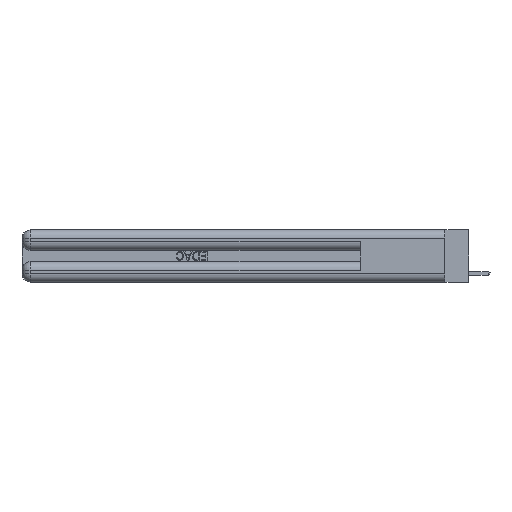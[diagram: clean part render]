
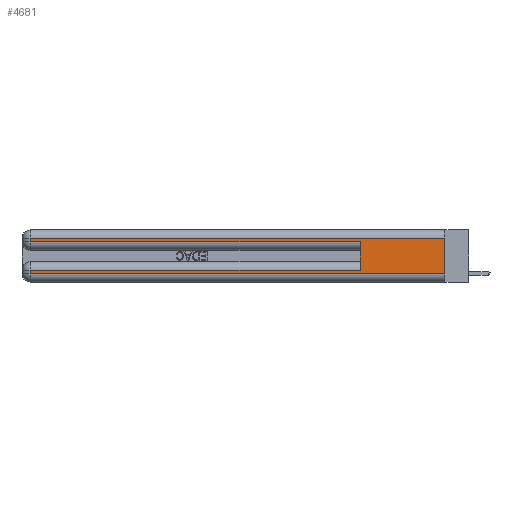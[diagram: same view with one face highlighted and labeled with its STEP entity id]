
A CAD part, left-side view. The second image highlights one B-rep face of the part: STEP entity #4681.
In plain terms, the highlighted planar face has unit normal (-1, 0, 0).
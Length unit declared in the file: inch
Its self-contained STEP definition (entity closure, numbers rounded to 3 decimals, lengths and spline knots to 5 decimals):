
#1505 = DIRECTION ( 'NONE',  ( 0., 0., -1. ) ) ;
#1712 = ORIENTED_EDGE ( 'NONE', *, *, #9419, .F. ) ;
#2761 = VECTOR ( 'NONE', #33430, 39.37008 ) ;
#2908 = DIRECTION ( 'NONE',  ( 0., 0., 1. ) ) ;
#3691 = EDGE_CURVE ( 'NONE', #10057, #9329, #4144, .T. ) ;
#4144 = LINE ( 'NONE', #16697, #21500 ) ;
#4260 = EDGE_CURVE ( 'NONE', #27985, #23001, #7281, .T. ) ;
#4681 = ADVANCED_FACE ( 'NONE', ( #18136 ), #33951, .F. ) ;
#5037 = ORIENTED_EDGE ( 'NONE', *, *, #18744, .T. ) ;
#5178 = ORIENTED_EDGE ( 'NONE', *, *, #24509, .F. ) ;
#6189 = LINE ( 'NONE', #11609, #26545 ) ;
#6500 = LINE ( 'NONE', #22339, #14391 ) ;
#7015 = AXIS2_PLACEMENT_3D ( 'NONE', #23599, #26409, #9858 ) ;
#7079 = DIRECTION ( 'NONE',  ( 0., -1., 0. ) ) ;
#7281 = LINE ( 'NONE', #24003, #27173 ) ;
#7609 = EDGE_CURVE ( 'NONE', #34385, #10057, #6500, .T. ) ;
#7647 = ORIENTED_EDGE ( 'NONE', *, *, #22046, .T. ) ;
#7881 = VECTOR ( 'NONE', #7079, 39.37008 ) ;
#9329 = VERTEX_POINT ( 'NONE', #12242 ) ;
#9419 = EDGE_CURVE ( 'NONE', #34385, #13860, #34396, .T. ) ;
#9858 = DIRECTION ( 'NONE',  ( 0., 0., -1. ) ) ;
#9875 = CARTESIAN_POINT ( 'NONE',  ( 0., 0., 0.06 ) ) ;
#9883 = CARTESIAN_POINT ( 'NONE',  ( 0., 2.94, 0.31 ) ) ;
#10057 = VERTEX_POINT ( 'NONE', #24075 ) ;
#10427 = DIRECTION ( 'NONE',  ( 0., 0., -1. ) ) ;
#11609 = CARTESIAN_POINT ( 'NONE',  ( 0., 0., 0.285 ) ) ;
#11956 = DIRECTION ( 'NONE',  ( 0., -1., 0. ) ) ;
#12094 = VERTEX_POINT ( 'NONE', #33825 ) ;
#12242 = CARTESIAN_POINT ( 'NONE',  ( 0., 2.94, 0.06 ) ) ;
#13860 = VERTEX_POINT ( 'NONE', #17883 ) ;
#14391 = VECTOR ( 'NONE', #33022, 39.37008 ) ;
#14629 = LINE ( 'NONE', #31311, #2761 ) ;
#15345 = LINE ( 'NONE', #20999, #15870 ) ;
#15870 = VECTOR ( 'NONE', #23285, 39.37008 ) ;
#16697 = CARTESIAN_POINT ( 'NONE',  ( 0., 2.94, 0.37 ) ) ;
#17404 = ORIENTED_EDGE ( 'NONE', *, *, #3691, .T. ) ;
#17883 = CARTESIAN_POINT ( 'NONE',  ( 0., 0.6, 0.285 ) ) ;
#18136 = FACE_OUTER_BOUND ( 'NONE', #26301, .T. ) ;
#18744 = EDGE_CURVE ( 'NONE', #12094, #27985, #14629, .T. ) ;
#18860 = ORIENTED_EDGE ( 'NONE', *, *, #34357, .T. ) ;
#19418 = CARTESIAN_POINT ( 'NONE',  ( 0., 0., 0.06 ) ) ;
#20696 = VECTOR ( 'NONE', #2908, 39.37008 ) ;
#20999 = CARTESIAN_POINT ( 'NONE',  ( 0., 0., 0.37 ) ) ;
#21500 = VECTOR ( 'NONE', #1505, 39.37008 ) ;
#22046 = EDGE_CURVE ( 'NONE', #9329, #27712, #34138, .T. ) ;
#22339 = CARTESIAN_POINT ( 'NONE',  ( 0., 0., 0.085 ) ) ;
#23001 = VERTEX_POINT ( 'NONE', #29271 ) ;
#23285 = DIRECTION ( 'NONE',  ( 0., 0., -1. ) ) ;
#23599 = CARTESIAN_POINT ( 'NONE',  ( 0., 0., 0.37 ) ) ;
#24003 = CARTESIAN_POINT ( 'NONE',  ( 0., 2.94, 0.37 ) ) ;
#24075 = CARTESIAN_POINT ( 'NONE',  ( 0., 2.94, 0.085 ) ) ;
#24509 = EDGE_CURVE ( 'NONE', #12094, #27712, #15345, .T. ) ;
#26301 = EDGE_LOOP ( 'NONE', ( #5178, #5037, #27346, #18860, #1712, #29734, #17404, #7647 ) ) ;
#26409 = DIRECTION ( 'NONE',  ( 1., 0., 0. ) ) ;
#26545 = VECTOR ( 'NONE', #11956, 39.37008 ) ;
#27173 = VECTOR ( 'NONE', #10427, 39.37008 ) ;
#27346 = ORIENTED_EDGE ( 'NONE', *, *, #4260, .T. ) ;
#27712 = VERTEX_POINT ( 'NONE', #19418 ) ;
#27985 = VERTEX_POINT ( 'NONE', #9883 ) ;
#29271 = CARTESIAN_POINT ( 'NONE',  ( 0., 2.94, 0.285 ) ) ;
#29476 = CARTESIAN_POINT ( 'NONE',  ( 0., 0.6, 0.145 ) ) ;
#29734 = ORIENTED_EDGE ( 'NONE', *, *, #7609, .T. ) ;
#31311 = CARTESIAN_POINT ( 'NONE',  ( 0., 0., 0.31 ) ) ;
#33022 = DIRECTION ( 'NONE',  ( 0., 1., 0. ) ) ;
#33050 = CARTESIAN_POINT ( 'NONE',  ( 0., 0.6, 0.085 ) ) ;
#33430 = DIRECTION ( 'NONE',  ( 0., 1., 0. ) ) ;
#33825 = CARTESIAN_POINT ( 'NONE',  ( 0., 0., 0.31 ) ) ;
#33951 = PLANE ( 'NONE',  #7015 ) ;
#34138 = LINE ( 'NONE', #9875, #7881 ) ;
#34357 = EDGE_CURVE ( 'NONE', #23001, #13860, #6189, .T. ) ;
#34385 = VERTEX_POINT ( 'NONE', #33050 ) ;
#34396 = LINE ( 'NONE', #29476, #20696 ) ;
